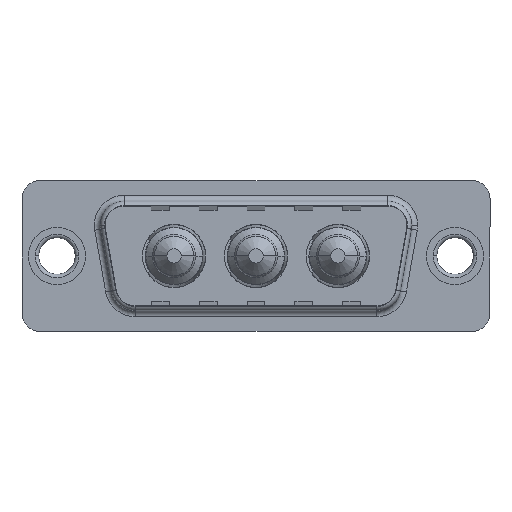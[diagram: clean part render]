
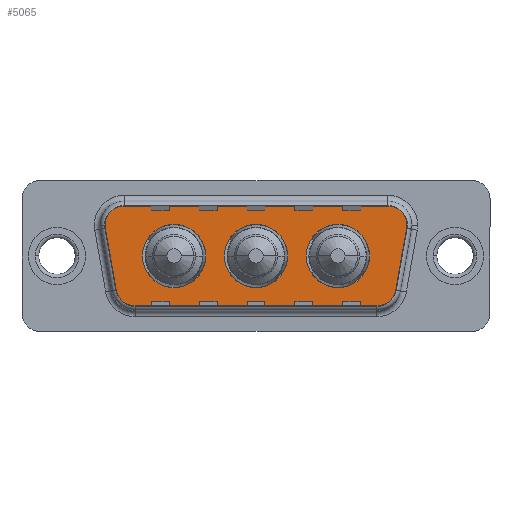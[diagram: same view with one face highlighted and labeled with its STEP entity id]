
A CAD part, top view. The second image highlights one B-rep face of the part: STEP entity #5065.
In plain terms, the highlighted planar face has unit normal (0, 0, 1).
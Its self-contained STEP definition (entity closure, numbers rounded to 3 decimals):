
#125 = LINE ( 'NONE', #7676, #6872 ) ;
#145 = VERTEX_POINT ( 'NONE', #5380 ) ;
#238 = VERTEX_POINT ( 'NONE', #1367 ) ;
#253 = AXIS2_PLACEMENT_3D ( 'NONE', #3855, #9791, #4708 ) ;
#361 = AXIS2_PLACEMENT_3D ( 'NONE', #2592, #8498, #3428 ) ;
#398 = CARTESIAN_POINT ( 'NONE',  ( 29.859, 2.553, 0. ) ) ;
#432 = CARTESIAN_POINT ( 'NONE',  ( 23.5, 0., 0. ) ) ;
#477 = CARTESIAN_POINT ( 'NONE',  ( 3.441, 2.553, 0. ) ) ;
#662 = AXIS2_PLACEMENT_3D ( 'NONE', #5046, #11016, #5960 ) ;
#698 = ORIENTED_EDGE ( 'NONE', *, *, #6975, .F. ) ;
#713 = VECTOR ( 'NONE', #10953, 1000. ) ;
#730 = EDGE_CURVE ( 'NONE', #2880, #1883, #4804, .T. ) ;
#764 = EDGE_CURVE ( 'NONE', #3265, #5039, #2308, .T. ) ;
#855 = CARTESIAN_POINT ( 'NONE',  ( 5.411, 4.9, 0. ) ) ;
#952 = VERTEX_POINT ( 'NONE', #1386 ) ;
#983 = FACE_BOUND ( 'NONE', #6529, .T. ) ;
#1022 = EDGE_LOOP ( 'NONE', ( #1380, #2254 ) ) ;
#1367 = CARTESIAN_POINT ( 'NONE',  ( 29.889, 2.9, 0. ) ) ;
#1380 = ORIENTED_EDGE ( 'NONE', *, *, #7396, .F. ) ;
#1386 = CARTESIAN_POINT ( 'NONE',  ( 27.889, 4.9, 0. ) ) ;
#1503 = CARTESIAN_POINT ( 'NONE',  ( 28.836, -3.247, 0. ) ) ;
#1531 = AXIS2_PLACEMENT_3D ( 'NONE', #10732, #10701, #10692 ) ;
#1561 = CIRCLE ( 'NONE', #361, 2. ) ;
#1641 = CARTESIAN_POINT ( 'NONE',  ( 27.889, 2.9, 0. ) ) ;
#1778 = DIRECTION ( 'NONE',  ( 0., 0., 1. ) ) ;
#1805 = EDGE_CURVE ( 'NONE', #952, #7775, #10864, .T. ) ;
#1883 = VERTEX_POINT ( 'NONE', #5934 ) ;
#1933 = PLANE ( 'NONE',  #4278 ) ;
#2038 = DIRECTION ( 'NONE',  ( 1., 0., 0. ) ) ;
#2053 = DIRECTION ( 'NONE',  ( 0., 0., 1. ) ) ;
#2084 = CARTESIAN_POINT ( 'NONE',  ( 14., 0., 0. ) ) ;
#2091 = CARTESIAN_POINT ( 'NONE',  ( 9.8, 0., 0. ) ) ;
#2254 = ORIENTED_EDGE ( 'NONE', *, *, #7617, .F. ) ;
#2308 = CIRCLE ( 'NONE', #10728, 2.65 ) ;
#2548 = DIRECTION ( 'NONE',  ( 1., 0., 0. ) ) ;
#2554 = DIRECTION ( 'NONE',  ( -1., 0., 0. ) ) ;
#2592 = CARTESIAN_POINT ( 'NONE',  ( 5.411, 2.9, 0. ) ) ;
#2748 = AXIS2_PLACEMENT_3D ( 'NONE', #2091, #2053, #2038 ) ;
#2880 = VERTEX_POINT ( 'NONE', #10312 ) ;
#2915 = EDGE_CURVE ( 'NONE', #9910, #9253, #4440, .T. ) ;
#2936 = CARTESIAN_POINT ( 'NONE',  ( 26.866, -2.9, 0. ) ) ;
#3005 = ORIENTED_EDGE ( 'NONE', *, *, #10554, .T. ) ;
#3031 = EDGE_CURVE ( 'NONE', #238, #952, #11123, .T. ) ;
#3102 = DIRECTION ( 'NONE',  ( 0., 0., 1. ) ) ;
#3265 = VERTEX_POINT ( 'NONE', #6151 ) ;
#3341 = ORIENTED_EDGE ( 'NONE', *, *, #10528, .T. ) ;
#3359 = EDGE_CURVE ( 'NONE', #8421, #9910, #9878, .T. ) ;
#3428 = DIRECTION ( 'NONE',  ( 1., 0., 0. ) ) ;
#3585 = CIRCLE ( 'NONE', #9808, 2. ) ;
#3690 = VERTEX_POINT ( 'NONE', #8858 ) ;
#3743 = CARTESIAN_POINT ( 'NONE',  ( 26.866, -4.9, 0. ) ) ;
#3855 = CARTESIAN_POINT ( 'NONE',  ( 16.65, 0., 0. ) ) ;
#4233 = DIRECTION ( 'NONE',  ( 1., 0., 0. ) ) ;
#4243 = ORIENTED_EDGE ( 'NONE', *, *, #6527, .T. ) ;
#4278 = AXIS2_PLACEMENT_3D ( 'NONE', #2936, #3102, #2548 ) ;
#4301 = CARTESIAN_POINT ( 'NONE',  ( 6.434, -2.9, 0. ) ) ;
#4372 = ORIENTED_EDGE ( 'NONE', *, *, #6848, .F. ) ;
#4375 = CIRCLE ( 'NONE', #2748, 2.65 ) ;
#4440 = LINE ( 'NONE', #398, #10145 ) ;
#4582 = EDGE_CURVE ( 'NONE', #1883, #8421, #125, .T. ) ;
#4701 = ORIENTED_EDGE ( 'NONE', *, *, #4582, .T. ) ;
#4708 = DIRECTION ( 'NONE',  ( 1., 0., 0. ) ) ;
#4709 = DIRECTION ( 'NONE',  ( 1., 0., 0. ) ) ;
#4804 = CIRCLE ( 'NONE', #9009, 2. ) ;
#4908 = CIRCLE ( 'NONE', #253, 2.65 ) ;
#5034 = CARTESIAN_POINT ( 'NONE',  ( 20.85, 0., 0. ) ) ;
#5039 = VERTEX_POINT ( 'NONE', #5034 ) ;
#5046 = CARTESIAN_POINT ( 'NONE',  ( 16.65, 0., 0. ) ) ;
#5058 = ORIENTED_EDGE ( 'NONE', *, *, #2915, .T. ) ;
#5065 = ADVANCED_FACE ( 'NONE', ( #5630, #983, #7860, #9841 ), #1933, .T. ) ;
#5182 = CARTESIAN_POINT ( 'NONE',  ( 19.3, 0., 0. ) ) ;
#5264 = DIRECTION ( 'NONE',  ( -1., 0., 0. ) ) ;
#5343 = LINE ( 'NONE', #477, #713 ) ;
#5380 = CARTESIAN_POINT ( 'NONE',  ( 3.441, 2.553, 0. ) ) ;
#5408 = DIRECTION ( 'NONE',  ( 0., 0., 1. ) ) ;
#5460 = CIRCLE ( 'NONE', #5946, 2.65 ) ;
#5630 = FACE_BOUND ( 'NONE', #1022, .T. ) ;
#5777 = ORIENTED_EDGE ( 'NONE', *, *, #3031, .T. ) ;
#5934 = CARTESIAN_POINT ( 'NONE',  ( 6.434, -4.9, 0. ) ) ;
#5946 = AXIS2_PLACEMENT_3D ( 'NONE', #6962, #1778, #7769 ) ;
#5960 = DIRECTION ( 'NONE',  ( 1., 0., 0. ) ) ;
#6045 = AXIS2_PLACEMENT_3D ( 'NONE', #6078, #5408, #5264 ) ;
#6078 = CARTESIAN_POINT ( 'NONE',  ( 27.889, 2.9, 0. ) ) ;
#6151 = CARTESIAN_POINT ( 'NONE',  ( 26.15, 0., 0. ) ) ;
#6527 = EDGE_CURVE ( 'NONE', #145, #2880, #5343, .T. ) ;
#6529 = EDGE_LOOP ( 'NONE', ( #6598, #9290 ) ) ;
#6585 = DIRECTION ( 'NONE',  ( 0.174, 0.985, 0. ) ) ;
#6598 = ORIENTED_EDGE ( 'NONE', *, *, #764, .F. ) ;
#6699 = CARTESIAN_POINT ( 'NONE',  ( 29.859, 2.553, 0. ) ) ;
#6848 = EDGE_CURVE ( 'NONE', #3690, #7943, #4375, .T. ) ;
#6872 = VECTOR ( 'NONE', #4709, 1000. ) ;
#6962 = CARTESIAN_POINT ( 'NONE',  ( 23.5, 0., 0. ) ) ;
#6975 = EDGE_CURVE ( 'NONE', #7943, #3690, #9819, .T. ) ;
#7396 = EDGE_CURVE ( 'NONE', #10618, #10796, #4908, .T. ) ;
#7479 = DIRECTION ( 'NONE',  ( -1., 0., 0. ) ) ;
#7617 = EDGE_CURVE ( 'NONE', #10796, #10618, #8478, .T. ) ;
#7655 = DIRECTION ( 'NONE',  ( 0., 0., 1. ) ) ;
#7676 = CARTESIAN_POINT ( 'NONE',  ( 6.434, -4.9, 0. ) ) ;
#7743 = EDGE_CURVE ( 'NONE', #5039, #3265, #5460, .T. ) ;
#7749 = DIRECTION ( 'NONE',  ( 0., 0., 1. ) ) ;
#7769 = DIRECTION ( 'NONE',  ( 1., 0., 0. ) ) ;
#7775 = VERTEX_POINT ( 'NONE', #855 ) ;
#7860 = FACE_BOUND ( 'NONE', #8539, .T. ) ;
#7943 = VERTEX_POINT ( 'NONE', #10562 ) ;
#8154 = EDGE_LOOP ( 'NONE', ( #8225, #5058, #3341, #5777, #8782, #3005, #4243, #9401, #4701 ) ) ;
#8225 = ORIENTED_EDGE ( 'NONE', *, *, #3359, .T. ) ;
#8421 = VERTEX_POINT ( 'NONE', #3743 ) ;
#8425 = AXIS2_PLACEMENT_3D ( 'NONE', #10500, #10420, #10390 ) ;
#8478 = CIRCLE ( 'NONE', #662, 2.65 ) ;
#8498 = DIRECTION ( 'NONE',  ( 0., 0., 1. ) ) ;
#8539 = EDGE_LOOP ( 'NONE', ( #698, #4372 ) ) ;
#8580 = VECTOR ( 'NONE', #7479, 1000. ) ;
#8782 = ORIENTED_EDGE ( 'NONE', *, *, #1805, .T. ) ;
#8858 = CARTESIAN_POINT ( 'NONE',  ( 7.15, 0., 0. ) ) ;
#9009 = AXIS2_PLACEMENT_3D ( 'NONE', #4301, #7749, #10548 ) ;
#9253 = VERTEX_POINT ( 'NONE', #6699 ) ;
#9283 = CARTESIAN_POINT ( 'NONE',  ( 5.411, 4.9, 0. ) ) ;
#9290 = ORIENTED_EDGE ( 'NONE', *, *, #7743, .F. ) ;
#9401 = ORIENTED_EDGE ( 'NONE', *, *, #730, .T. ) ;
#9765 = DIRECTION ( 'NONE',  ( 0., 0., 1. ) ) ;
#9791 = DIRECTION ( 'NONE',  ( 0., 0., 1. ) ) ;
#9808 = AXIS2_PLACEMENT_3D ( 'NONE', #1641, #7655, #2554 ) ;
#9819 = CIRCLE ( 'NONE', #8425, 2.65 ) ;
#9841 = FACE_OUTER_BOUND ( 'NONE', #8154, .T. ) ;
#9878 = CIRCLE ( 'NONE', #1531, 2. ) ;
#9910 = VERTEX_POINT ( 'NONE', #1503 ) ;
#10145 = VECTOR ( 'NONE', #6585, 1000. ) ;
#10312 = CARTESIAN_POINT ( 'NONE',  ( 4.464, -3.247, 0. ) ) ;
#10390 = DIRECTION ( 'NONE',  ( 1., 0., 0. ) ) ;
#10420 = DIRECTION ( 'NONE',  ( 0., 0., 1. ) ) ;
#10500 = CARTESIAN_POINT ( 'NONE',  ( 9.8, 0., 0. ) ) ;
#10528 = EDGE_CURVE ( 'NONE', #9253, #238, #3585, .T. ) ;
#10548 = DIRECTION ( 'NONE',  ( -1., 0., 0. ) ) ;
#10554 = EDGE_CURVE ( 'NONE', #7775, #145, #1561, .T. ) ;
#10562 = CARTESIAN_POINT ( 'NONE',  ( 12.45, 0., 0. ) ) ;
#10618 = VERTEX_POINT ( 'NONE', #5182 ) ;
#10692 = DIRECTION ( 'NONE',  ( 1., 0., 0. ) ) ;
#10701 = DIRECTION ( 'NONE',  ( 0., 0., 1. ) ) ;
#10728 = AXIS2_PLACEMENT_3D ( 'NONE', #432, #9765, #4233 ) ;
#10732 = CARTESIAN_POINT ( 'NONE',  ( 26.866, -2.9, 0. ) ) ;
#10796 = VERTEX_POINT ( 'NONE', #2084 ) ;
#10864 = LINE ( 'NONE', #9283, #8580 ) ;
#10953 = DIRECTION ( 'NONE',  ( 0.174, -0.985, 0. ) ) ;
#11016 = DIRECTION ( 'NONE',  ( 0., 0., 1. ) ) ;
#11123 = CIRCLE ( 'NONE', #6045, 2. ) ;
